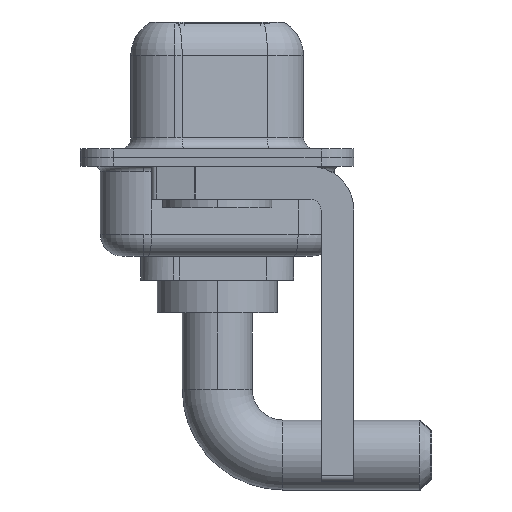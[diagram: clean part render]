
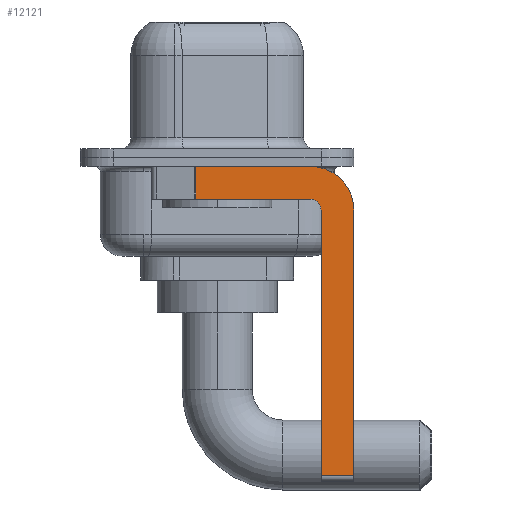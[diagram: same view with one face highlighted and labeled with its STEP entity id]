
A CAD part, left-side view. The second image highlights one B-rep face of the part: STEP entity #12121.
In plain terms, the highlighted planar face has unit normal (-1, 0, 0).
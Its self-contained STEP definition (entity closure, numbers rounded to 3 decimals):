
#7 = CARTESIAN_POINT ( 'NONE',  ( -2.9, -6.25, -2.4 ) ) ;
#137 = EDGE_LOOP ( 'NONE', ( #11611, #2777, #10534, #1385, #11084, #13623, #949, #10272 ) ) ;
#483 = VECTOR ( 'NONE', #5758, 1000. ) ;
#521 = LINE ( 'NONE', #7354, #1870 ) ;
#526 = DIRECTION ( 'NONE',  ( 0., 1., 0. ) ) ;
#760 = CARTESIAN_POINT ( 'NONE',  ( -2.9, -4.25, -14.55 ) ) ;
#949 = ORIENTED_EDGE ( 'NONE', *, *, #8326, .F. ) ;
#1227 = CARTESIAN_POINT ( 'NONE',  ( -2.9, 0.978, -1.9 ) ) ;
#1385 = ORIENTED_EDGE ( 'NONE', *, *, #12870, .F. ) ;
#1443 = AXIS2_PLACEMENT_3D ( 'NONE', #6983, #4780, #12506 ) ;
#1704 = AXIS2_PLACEMENT_3D ( 'NONE', #6273, #7355, #2659 ) ;
#1870 = VECTOR ( 'NONE', #7431, 1000. ) ;
#2548 = DIRECTION ( 'NONE',  ( 1., 0., 0. ) ) ;
#2659 = DIRECTION ( 'NONE',  ( 0., 0., -1. ) ) ;
#2777 = ORIENTED_EDGE ( 'NONE', *, *, #7140, .T. ) ;
#2902 = DIRECTION ( 'NONE',  ( 0., 0., 1. ) ) ;
#2907 = EDGE_CURVE ( 'NONE', #8132, #9095, #4012, .T. ) ;
#3510 = CARTESIAN_POINT ( 'NONE',  ( -2.9, -4.25, -2.4 ) ) ;
#3536 = LINE ( 'NONE', #7, #483 ) ;
#4012 = LINE ( 'NONE', #11882, #5579 ) ;
#4350 = VERTEX_POINT ( 'NONE', #6194 ) ;
#4780 = DIRECTION ( 'NONE',  ( -1., 0., 0. ) ) ;
#5219 = EDGE_CURVE ( 'NONE', #8132, #4350, #6212, .T. ) ;
#5579 = VECTOR ( 'NONE', #2902, 1000. ) ;
#5758 = DIRECTION ( 'NONE',  ( 0., 0., -1. ) ) ;
#5970 = CARTESIAN_POINT ( 'NONE',  ( -2.9, 0.978, -0.4 ) ) ;
#6194 = CARTESIAN_POINT ( 'NONE',  ( -2.9, -6.25, -14.55 ) ) ;
#6212 = LINE ( 'NONE', #760, #9109 ) ;
#6273 = CARTESIAN_POINT ( 'NONE',  ( -2.9, -4.25, -2.4 ) ) ;
#6591 = VERTEX_POINT ( 'NONE', #11308 ) ;
#6738 = CARTESIAN_POINT ( 'NONE',  ( -2.9, 3., -0.4 ) ) ;
#6983 = CARTESIAN_POINT ( 'NONE',  ( -2.9, -4.25, -2.4 ) ) ;
#7140 = EDGE_CURVE ( 'NONE', #11107, #7964, #521, .T. ) ;
#7354 = CARTESIAN_POINT ( 'NONE',  ( -2.9, 0.978, -1.9 ) ) ;
#7355 = DIRECTION ( 'NONE',  ( 1., 0., 0. ) ) ;
#7431 = DIRECTION ( 'NONE',  ( 0., 0., -1. ) ) ;
#7906 = EDGE_CURVE ( 'NONE', #12510, #6591, #8461, .T. ) ;
#7964 = VERTEX_POINT ( 'NONE', #1227 ) ;
#8112 = CARTESIAN_POINT ( 'NONE',  ( -2.9, -4.25, -0.4 ) ) ;
#8132 = VERTEX_POINT ( 'NONE', #11665 ) ;
#8326 = EDGE_CURVE ( 'NONE', #6591, #4350, #3536, .T. ) ;
#8461 = CIRCLE ( 'NONE', #12238, 2. ) ;
#8468 = LINE ( 'NONE', #12963, #14170 ) ;
#8784 = EDGE_CURVE ( 'NONE', #11107, #12510, #13504, .T. ) ;
#8952 = DIRECTION ( 'NONE',  ( 0., 0., -1. ) ) ;
#9095 = VERTEX_POINT ( 'NONE', #14144 ) ;
#9109 = VECTOR ( 'NONE', #10689, 1000. ) ;
#10140 = CIRCLE ( 'NONE', #1443, 0.5 ) ;
#10272 = ORIENTED_EDGE ( 'NONE', *, *, #7906, .F. ) ;
#10534 = ORIENTED_EDGE ( 'NONE', *, *, #10798, .F. ) ;
#10607 = FACE_OUTER_BOUND ( 'NONE', #137, .T. ) ;
#10689 = DIRECTION ( 'NONE',  ( 0., -1., 0. ) ) ;
#10798 = EDGE_CURVE ( 'NONE', #11021, #7964, #8468, .T. ) ;
#11021 = VERTEX_POINT ( 'NONE', #12936 ) ;
#11084 = ORIENTED_EDGE ( 'NONE', *, *, #2907, .F. ) ;
#11107 = VERTEX_POINT ( 'NONE', #5970 ) ;
#11223 = DIRECTION ( 'NONE',  ( 0., -1., 0. ) ) ;
#11308 = CARTESIAN_POINT ( 'NONE',  ( -2.9, -6.25, -2.4 ) ) ;
#11611 = ORIENTED_EDGE ( 'NONE', *, *, #8784, .F. ) ;
#11665 = CARTESIAN_POINT ( 'NONE',  ( -2.9, -4.75, -14.55 ) ) ;
#11790 = PLANE ( 'NONE',  #1704 ) ;
#11882 = CARTESIAN_POINT ( 'NONE',  ( -2.9, -4.75, -14.8 ) ) ;
#12023 = VECTOR ( 'NONE', #11223, 1000. ) ;
#12121 = ADVANCED_FACE ( 'NONE', ( #10607 ), #11790, .F. ) ;
#12238 = AXIS2_PLACEMENT_3D ( 'NONE', #3510, #2548, #8952 ) ;
#12506 = DIRECTION ( 'NONE',  ( 0., 0., 1. ) ) ;
#12510 = VERTEX_POINT ( 'NONE', #8112 ) ;
#12870 = EDGE_CURVE ( 'NONE', #9095, #11021, #10140, .T. ) ;
#12936 = CARTESIAN_POINT ( 'NONE',  ( -2.9, -4.25, -1.9 ) ) ;
#12963 = CARTESIAN_POINT ( 'NONE',  ( -2.9, -4.25, -1.9 ) ) ;
#13504 = LINE ( 'NONE', #6738, #12023 ) ;
#13623 = ORIENTED_EDGE ( 'NONE', *, *, #5219, .T. ) ;
#14144 = CARTESIAN_POINT ( 'NONE',  ( -2.9, -4.75, -2.4 ) ) ;
#14170 = VECTOR ( 'NONE', #526, 1000. ) ;
